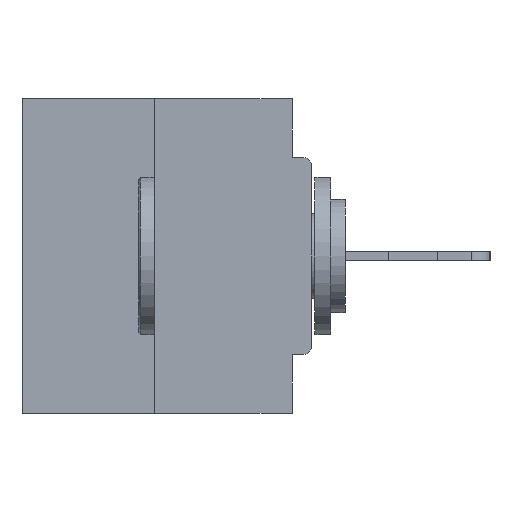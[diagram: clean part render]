
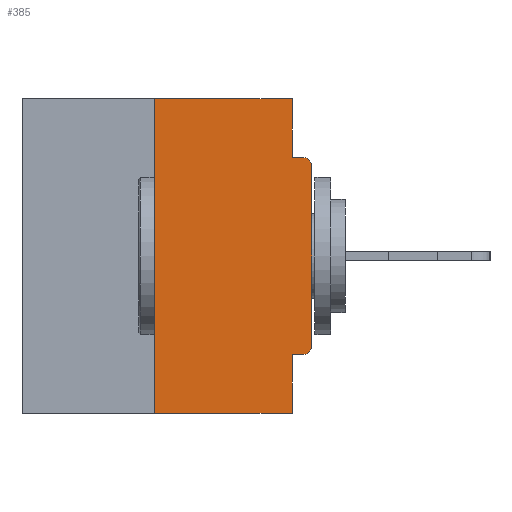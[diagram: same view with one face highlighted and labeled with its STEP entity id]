
A CAD part, left-side view. The second image highlights one B-rep face of the part: STEP entity #385.
In plain terms, the highlighted planar face has unit normal (-1, 0, 0).
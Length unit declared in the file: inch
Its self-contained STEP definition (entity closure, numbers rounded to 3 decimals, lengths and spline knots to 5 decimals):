
#314 = CARTESIAN_POINT ( 'NONE',  ( 0., 0., -0.1085 ) ) ;
#385 = ADVANCED_FACE ( 'NONE', ( #14949 ), #12778, .F. ) ;
#1113 = DIRECTION ( 'NONE',  ( 0., 0., -1. ) ) ;
#1262 = ORIENTED_EDGE ( 'NONE', *, *, #30185, .F. ) ;
#1388 = EDGE_CURVE ( 'NONE', #3003, #1992, #29206, .T. ) ;
#1992 = VERTEX_POINT ( 'NONE', #314 ) ;
#2757 = AXIS2_PLACEMENT_3D ( 'NONE', #30618, #5194, #7744 ) ;
#2826 = DIRECTION ( 'NONE',  ( 0., 0., -1. ) ) ;
#3003 = VERTEX_POINT ( 'NONE', #16307 ) ;
#3036 = CARTESIAN_POINT ( 'NONE',  ( 0., 0.25, 0. ) ) ;
#3055 = CARTESIAN_POINT ( 'NONE',  ( 0., 0.031, -0.4065 ) ) ;
#3252 = VECTOR ( 'NONE', #11278, 39.37008 ) ;
#3874 = CARTESIAN_POINT ( 'NONE',  ( 0., 0.031, 0. ) ) ;
#3975 = VERTEX_POINT ( 'NONE', #27945 ) ;
#4636 = VECTOR ( 'NONE', #2826, 39.37008 ) ;
#5194 = DIRECTION ( 'NONE',  ( 1., 0., 0. ) ) ;
#5418 = VERTEX_POINT ( 'NONE', #3055 ) ;
#6217 = DIRECTION ( 'NONE',  ( 0., -1., 0. ) ) ;
#6853 = ORIENTED_EDGE ( 'NONE', *, *, #7967, .T. ) ;
#7152 = ORIENTED_EDGE ( 'NONE', *, *, #29368, .F. ) ;
#7608 = LINE ( 'NONE', #16156, #24782 ) ;
#7744 = DIRECTION ( 'NONE',  ( 0., 0., -1. ) ) ;
#7882 = ORIENTED_EDGE ( 'NONE', *, *, #30921, .F. ) ;
#7967 = EDGE_CURVE ( 'NONE', #23786, #3003, #22948, .T. ) ;
#8653 = LINE ( 'NONE', #22412, #16613 ) ;
#8747 = DIRECTION ( 'NONE',  ( -1., 0., 0. ) ) ;
#9974 = EDGE_LOOP ( 'NONE', ( #7882, #16567, #12507, #23814, #7152, #6853, #12159, #11517, #1262, #24605 ) ) ;
#9975 = VECTOR ( 'NONE', #26437, 39.37008 ) ;
#10066 = VERTEX_POINT ( 'NONE', #23134 ) ;
#10431 = CARTESIAN_POINT ( 'NONE',  ( 0., 0.015, -0.1085 ) ) ;
#10741 = CIRCLE ( 'NONE', #15984, 0.015 ) ;
#10965 = CARTESIAN_POINT ( 'NONE',  ( 0., 0.015, -0.3915 ) ) ;
#11125 = CARTESIAN_POINT ( 'NONE',  ( 0., 0.25, 0. ) ) ;
#11278 = DIRECTION ( 'NONE',  ( 0., 0., 1. ) ) ;
#11517 = ORIENTED_EDGE ( 'NONE', *, *, #30701, .T. ) ;
#12159 = ORIENTED_EDGE ( 'NONE', *, *, #1388, .T. ) ;
#12507 = ORIENTED_EDGE ( 'NONE', *, *, #17311, .T. ) ;
#12778 = PLANE ( 'NONE',  #2757 ) ;
#14576 = DIRECTION ( 'NONE',  ( 0., -1., 0. ) ) ;
#14949 = FACE_OUTER_BOUND ( 'NONE', #9974, .T. ) ;
#15984 = AXIS2_PLACEMENT_3D ( 'NONE', #10431, #28289, #30848 ) ;
#16156 = CARTESIAN_POINT ( 'NONE',  ( 0., 0., -0.4065 ) ) ;
#16192 = VERTEX_POINT ( 'NONE', #23747 ) ;
#16307 = CARTESIAN_POINT ( 'NONE',  ( 0., 0., -0.3915 ) ) ;
#16367 = LINE ( 'NONE', #18865, #9975 ) ;
#16567 = ORIENTED_EDGE ( 'NONE', *, *, #29615, .F. ) ;
#16613 = VECTOR ( 'NONE', #14576, 39.37008 ) ;
#16815 = VECTOR ( 'NONE', #21021, 39.37008 ) ;
#17311 = EDGE_CURVE ( 'NONE', #23626, #10066, #8653, .T. ) ;
#17555 = VECTOR ( 'NONE', #6217, 39.37008 ) ;
#18425 = LINE ( 'NONE', #3036, #16815 ) ;
#18728 = DIRECTION ( 'NONE',  ( 0., 1., 0. ) ) ;
#18865 = CARTESIAN_POINT ( 'NONE',  ( 0., 0.46, 0. ) ) ;
#21021 = DIRECTION ( 'NONE',  ( 0., 0., 1. ) ) ;
#21559 = VERTEX_POINT ( 'NONE', #3874 ) ;
#21886 = VERTEX_POINT ( 'NONE', #11125 ) ;
#22412 = CARTESIAN_POINT ( 'NONE',  ( 0., 0.46, -0.5 ) ) ;
#22948 = CIRCLE ( 'NONE', #28991, 0.015 ) ;
#23134 = CARTESIAN_POINT ( 'NONE',  ( 0., 0.031, -0.5 ) ) ;
#23451 = CARTESIAN_POINT ( 'NONE',  ( 0., 0.25, -0.5 ) ) ;
#23481 = CARTESIAN_POINT ( 'NONE',  ( 0., 0.031, 0. ) ) ;
#23626 = VERTEX_POINT ( 'NONE', #23451 ) ;
#23747 = CARTESIAN_POINT ( 'NONE',  ( 0., 0.015, -0.0935 ) ) ;
#23786 = VERTEX_POINT ( 'NONE', #29548 ) ;
#23814 = ORIENTED_EDGE ( 'NONE', *, *, #28715, .F. ) ;
#23882 = CARTESIAN_POINT ( 'NONE',  ( 0., 0., -0.0935 ) ) ;
#24605 = ORIENTED_EDGE ( 'NONE', *, *, #25202, .F. ) ;
#24782 = VECTOR ( 'NONE', #18728, 39.37008 ) ;
#25202 = EDGE_CURVE ( 'NONE', #21559, #3975, #25818, .T. ) ;
#25818 = LINE ( 'NONE', #23481, #4636 ) ;
#25934 = LINE ( 'NONE', #23882, #17555 ) ;
#26437 = DIRECTION ( 'NONE',  ( 0., -1., 0. ) ) ;
#26563 = CARTESIAN_POINT ( 'NONE',  ( 0., 0., 0. ) ) ;
#27636 = VECTOR ( 'NONE', #32085, 39.37008 ) ;
#27945 = CARTESIAN_POINT ( 'NONE',  ( 0., 0.031, -0.0935 ) ) ;
#28289 = DIRECTION ( 'NONE',  ( -1., 0., 0. ) ) ;
#28715 = EDGE_CURVE ( 'NONE', #5418, #10066, #31242, .T. ) ;
#28991 = AXIS2_PLACEMENT_3D ( 'NONE', #10965, #8747, #1113 ) ;
#29206 = LINE ( 'NONE', #26563, #3252 ) ;
#29368 = EDGE_CURVE ( 'NONE', #23786, #5418, #7608, .T. ) ;
#29548 = CARTESIAN_POINT ( 'NONE',  ( 0., 0.015, -0.4065 ) ) ;
#29615 = EDGE_CURVE ( 'NONE', #23626, #21886, #18425, .T. ) ;
#30185 = EDGE_CURVE ( 'NONE', #3975, #16192, #25934, .T. ) ;
#30618 = CARTESIAN_POINT ( 'NONE',  ( 0., 0.46, 0. ) ) ;
#30701 = EDGE_CURVE ( 'NONE', #1992, #16192, #10741, .T. ) ;
#30848 = DIRECTION ( 'NONE',  ( 0., 0., -1. ) ) ;
#30921 = EDGE_CURVE ( 'NONE', #21886, #21559, #16367, .T. ) ;
#31242 = LINE ( 'NONE', #32301, #27636 ) ;
#32085 = DIRECTION ( 'NONE',  ( 0., 0., -1. ) ) ;
#32301 = CARTESIAN_POINT ( 'NONE',  ( 0., 0.031, -0.5 ) ) ;
